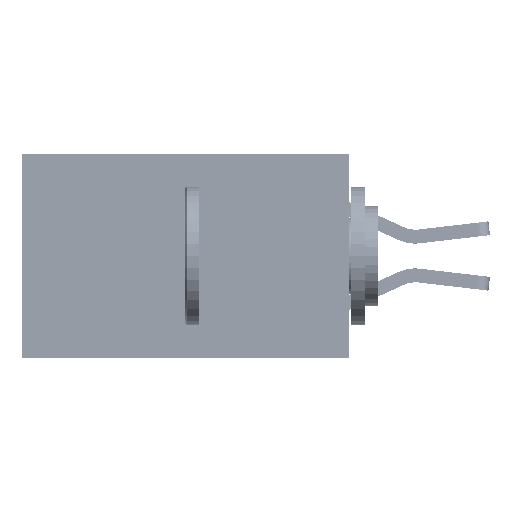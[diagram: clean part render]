
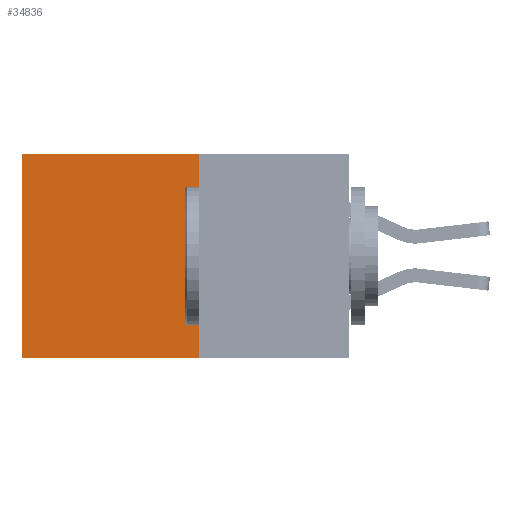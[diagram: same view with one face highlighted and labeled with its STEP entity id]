
A CAD part, left-side view. The second image highlights one B-rep face of the part: STEP entity #34836.
In plain terms, the highlighted planar face has unit normal (-1, 0, 0).
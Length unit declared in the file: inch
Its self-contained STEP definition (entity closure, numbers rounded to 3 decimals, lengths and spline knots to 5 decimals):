
#400 = VERTEX_POINT ( 'NONE', #23754 ) ;
#896 = AXIS2_PLACEMENT_3D ( 'NONE', #31164, #3311, #22909 ) ;
#1460 = VERTEX_POINT ( 'NONE', #23085 ) ;
#1588 = CARTESIAN_POINT ( 'NONE',  ( 0.277, 0.27, 0. ) ) ;
#3311 = DIRECTION ( 'NONE',  ( 1., 0., 0. ) ) ;
#6550 = DIRECTION ( 'NONE',  ( 0., 1., 0. ) ) ;
#7117 = VECTOR ( 'NONE', #6550, 39.37008 ) ;
#7327 = EDGE_CURVE ( 'NONE', #400, #14100, #13416, .T. ) ;
#9363 = CARTESIAN_POINT ( 'NONE',  ( 0.277, 0.27, -0.37 ) ) ;
#9761 = LINE ( 'NONE', #9363, #7117 ) ;
#10079 = ORIENTED_EDGE ( 'NONE', *, *, #15113, .T. ) ;
#10544 = LINE ( 'NONE', #18969, #28798 ) ;
#10607 = ORIENTED_EDGE ( 'NONE', *, *, #7327, .F. ) ;
#12316 = VECTOR ( 'NONE', #29554, 39.37008 ) ;
#13293 = CARTESIAN_POINT ( 'NONE',  ( 0.277, 0.59, 0. ) ) ;
#13416 = LINE ( 'NONE', #23365, #34748 ) ;
#14100 = VERTEX_POINT ( 'NONE', #14901 ) ;
#14901 = CARTESIAN_POINT ( 'NONE',  ( 0.277, 0.27, -0.37 ) ) ;
#15113 = EDGE_CURVE ( 'NONE', #400, #34527, #19283, .T. ) ;
#18969 = CARTESIAN_POINT ( 'NONE',  ( 0.277, 0.59, -0.37 ) ) ;
#19283 = LINE ( 'NONE', #1588, #12316 ) ;
#20033 = PLANE ( 'NONE',  #896 ) ;
#22909 = DIRECTION ( 'NONE',  ( 0., 0., -1. ) ) ;
#23085 = CARTESIAN_POINT ( 'NONE',  ( 0.277, 0.59, -0.37 ) ) ;
#23365 = CARTESIAN_POINT ( 'NONE',  ( 0.277, 0.27, -0.37 ) ) ;
#23754 = CARTESIAN_POINT ( 'NONE',  ( 0.277, 0.27, 0. ) ) ;
#28798 = VECTOR ( 'NONE', #35706, 39.37008 ) ;
#29554 = DIRECTION ( 'NONE',  ( 0., 1., 0. ) ) ;
#31164 = CARTESIAN_POINT ( 'NONE',  ( 0.277, 0.27, -0.37 ) ) ;
#31742 = DIRECTION ( 'NONE',  ( 0., 0., -1. ) ) ;
#31776 = EDGE_LOOP ( 'NONE', ( #33338, #33257, #10607, #10079 ) ) ;
#31960 = FACE_OUTER_BOUND ( 'NONE', #31776, .T. ) ;
#33257 = ORIENTED_EDGE ( 'NONE', *, *, #33432, .F. ) ;
#33338 = ORIENTED_EDGE ( 'NONE', *, *, #36014, .T. ) ;
#33432 = EDGE_CURVE ( 'NONE', #14100, #1460, #9761, .T. ) ;
#34527 = VERTEX_POINT ( 'NONE', #13293 ) ;
#34748 = VECTOR ( 'NONE', #31742, 39.37008 ) ;
#34836 = ADVANCED_FACE ( 'NONE', ( #31960 ), #20033, .F. ) ;
#35706 = DIRECTION ( 'NONE',  ( 0., 0., -1. ) ) ;
#36014 = EDGE_CURVE ( 'NONE', #34527, #1460, #10544, .T. ) ;
